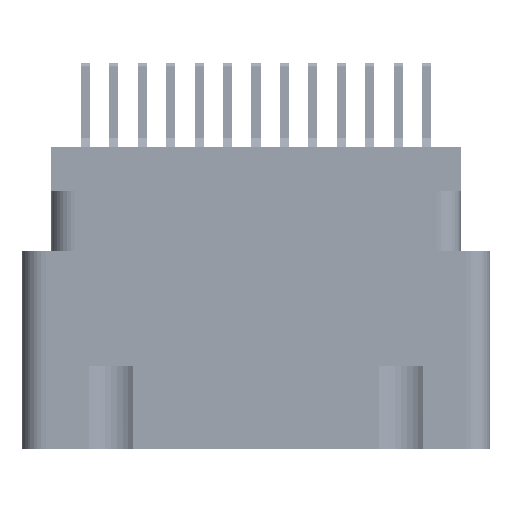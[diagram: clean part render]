
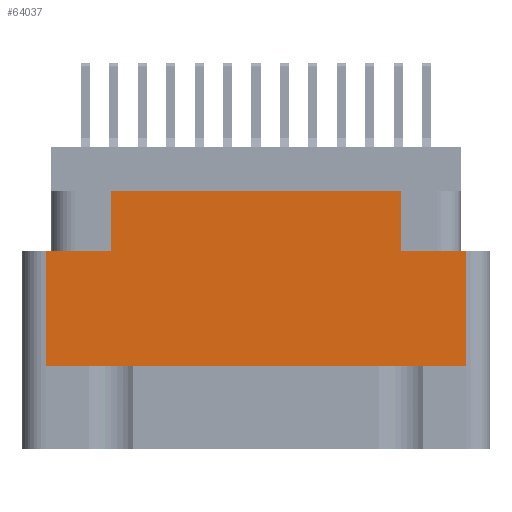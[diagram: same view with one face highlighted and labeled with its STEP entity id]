
A CAD part, left-side view. The second image highlights one B-rep face of the part: STEP entity #64037.
In plain terms, the highlighted planar face has unit normal (-1, 0, 0).
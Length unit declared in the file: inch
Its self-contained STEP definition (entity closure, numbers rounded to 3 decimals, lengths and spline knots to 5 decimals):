
#1434 = DIRECTION ( 'NONE',  ( 0., -1., 0. ) ) ;
#2203 = PLANE ( 'NONE',  #55045 ) ;
#3494 = VERTEX_POINT ( 'NONE', #37945 ) ;
#3522 = LINE ( 'NONE', #62195, #60479 ) ;
#4025 = EDGE_CURVE ( 'NONE', #10604, #38786, #34011, .T. ) ;
#5696 = VECTOR ( 'NONE', #68572, 39.37008 ) ;
#8331 = LINE ( 'NONE', #31240, #35931 ) ;
#10604 = VERTEX_POINT ( 'NONE', #27637 ) ;
#13515 = CARTESIAN_POINT ( 'NONE',  ( -1.359, -0.3825, -0.274 ) ) ;
#14457 = EDGE_CURVE ( 'NONE', #38786, #3494, #19204, .T. ) ;
#14677 = CARTESIAN_POINT ( 'NONE',  ( -1.359, 0.3825, -0.274 ) ) ;
#16063 = EDGE_CURVE ( 'NONE', #38313, #60543, #25655, .T. ) ;
#18077 = VERTEX_POINT ( 'NONE', #63312 ) ;
#19204 = LINE ( 'NONE', #39253, #56316 ) ;
#21194 = CARTESIAN_POINT ( 'NONE',  ( -1.359, 0., -0.578 ) ) ;
#22398 = EDGE_CURVE ( 'NONE', #60543, #46953, #8331, .T. ) ;
#22846 = VECTOR ( 'NONE', #46849, 39.37008 ) ;
#23334 = EDGE_CURVE ( 'NONE', #18077, #10604, #64488, .T. ) ;
#25655 = LINE ( 'NONE', #21194, #37660 ) ;
#26820 = CARTESIAN_POINT ( 'NONE',  ( -1.359, -0.555, -0.274 ) ) ;
#27411 = CARTESIAN_POINT ( 'NONE',  ( -1.359, 0.555, -0.578 ) ) ;
#27444 = ORIENTED_EDGE ( 'NONE', *, *, #43954, .F. ) ;
#27637 = CARTESIAN_POINT ( 'NONE',  ( -1.359, 0.3825, -0.274 ) ) ;
#29282 = VERTEX_POINT ( 'NONE', #62804 ) ;
#30780 = DIRECTION ( 'NONE',  ( 0., 0., 1. ) ) ;
#31240 = CARTESIAN_POINT ( 'NONE',  ( -1.359, -0.555, -0.798 ) ) ;
#33480 = VECTOR ( 'NONE', #58677, 39.37008 ) ;
#34011 = LINE ( 'NONE', #14677, #57363 ) ;
#34327 = EDGE_CURVE ( 'NONE', #18077, #38313, #3522, .T. ) ;
#35652 = DIRECTION ( 'NONE',  ( -1., 0., 0. ) ) ;
#35852 = DIRECTION ( 'NONE',  ( 0., 0., -1. ) ) ;
#35931 = VECTOR ( 'NONE', #30780, 39.37008 ) ;
#36236 = CARTESIAN_POINT ( 'NONE',  ( -1.359, 0., -0.274 ) ) ;
#37344 = ORIENTED_EDGE ( 'NONE', *, *, #39039, .T. ) ;
#37660 = VECTOR ( 'NONE', #65936, 39.37008 ) ;
#37945 = CARTESIAN_POINT ( 'NONE',  ( -1.359, -0.3825, -0.117 ) ) ;
#38313 = VERTEX_POINT ( 'NONE', #27411 ) ;
#38786 = VERTEX_POINT ( 'NONE', #44672 ) ;
#39039 = EDGE_CURVE ( 'NONE', #29282, #3494, #54782, .T. ) ;
#39253 = CARTESIAN_POINT ( 'NONE',  ( -1.359, 0.617, -0.117 ) ) ;
#41729 = ORIENTED_EDGE ( 'NONE', *, *, #22398, .T. ) ;
#43954 = EDGE_CURVE ( 'NONE', #29282, #46953, #49031, .T. ) ;
#44672 = CARTESIAN_POINT ( 'NONE',  ( -1.359, 0.3825, -0.117 ) ) ;
#45541 = ORIENTED_EDGE ( 'NONE', *, *, #14457, .F. ) ;
#46295 = DIRECTION ( 'NONE',  ( 0., 0., 1. ) ) ;
#46849 = DIRECTION ( 'NONE',  ( 0., 0., 1. ) ) ;
#46953 = VERTEX_POINT ( 'NONE', #26820 ) ;
#47036 = DIRECTION ( 'NONE',  ( 0., 0., 1. ) ) ;
#47130 = ORIENTED_EDGE ( 'NONE', *, *, #23334, .F. ) ;
#49031 = LINE ( 'NONE', #36236, #33480 ) ;
#52894 = EDGE_LOOP ( 'NONE', ( #47130, #55635, #59337, #41729, #27444, #37344, #45541, #65603 ) ) ;
#53316 = FACE_OUTER_BOUND ( 'NONE', #52894, .T. ) ;
#54782 = LINE ( 'NONE', #13515, #22846 ) ;
#55045 = AXIS2_PLACEMENT_3D ( 'NONE', #68582, #35652, #46295 ) ;
#55635 = ORIENTED_EDGE ( 'NONE', *, *, #34327, .T. ) ;
#56316 = VECTOR ( 'NONE', #1434, 39.37008 ) ;
#57363 = VECTOR ( 'NONE', #47036, 39.37008 ) ;
#57936 = CARTESIAN_POINT ( 'NONE',  ( -1.359, -0.555, -0.578 ) ) ;
#58677 = DIRECTION ( 'NONE',  ( 0., -1., 0. ) ) ;
#59337 = ORIENTED_EDGE ( 'NONE', *, *, #16063, .T. ) ;
#60479 = VECTOR ( 'NONE', #35852, 39.37008 ) ;
#60543 = VERTEX_POINT ( 'NONE', #57936 ) ;
#62195 = CARTESIAN_POINT ( 'NONE',  ( -1.359, 0.555, -0.798 ) ) ;
#62804 = CARTESIAN_POINT ( 'NONE',  ( -1.359, -0.3825, -0.274 ) ) ;
#63205 = CARTESIAN_POINT ( 'NONE',  ( -1.359, 0., -0.274 ) ) ;
#63312 = CARTESIAN_POINT ( 'NONE',  ( -1.359, 0.555, -0.274 ) ) ;
#64037 = ADVANCED_FACE ( 'NONE', ( #53316 ), #2203, .T. ) ;
#64488 = LINE ( 'NONE', #63205, #5696 ) ;
#65603 = ORIENTED_EDGE ( 'NONE', *, *, #4025, .F. ) ;
#65936 = DIRECTION ( 'NONE',  ( 0., -1., 0. ) ) ;
#68572 = DIRECTION ( 'NONE',  ( 0., -1., 0. ) ) ;
#68582 = CARTESIAN_POINT ( 'NONE',  ( -1.359, -0.617, -0.798 ) ) ;
